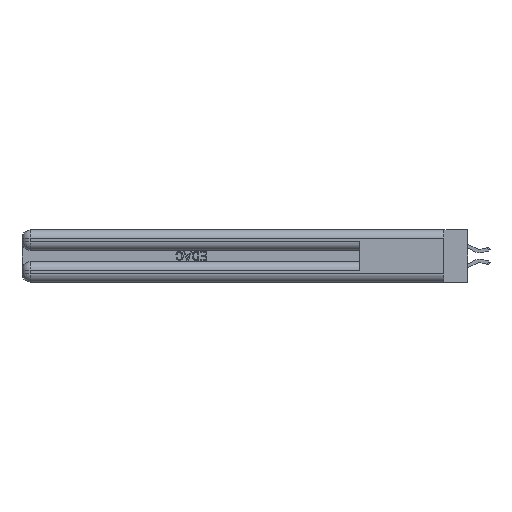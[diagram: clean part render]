
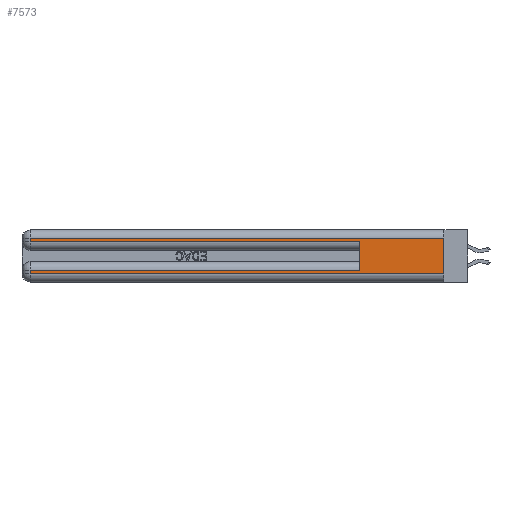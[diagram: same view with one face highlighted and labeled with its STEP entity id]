
A CAD part, left-side view. The second image highlights one B-rep face of the part: STEP entity #7573.
In plain terms, the highlighted planar face has unit normal (-1, 0, 0).
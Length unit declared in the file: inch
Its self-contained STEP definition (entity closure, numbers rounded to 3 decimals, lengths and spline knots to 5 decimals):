
#94 = ORIENTED_EDGE ( 'NONE', *, *, #21787, .T. ) ;
#700 = LINE ( 'NONE', #4594, #24358 ) ;
#827 = VECTOR ( 'NONE', #29109, 39.37008 ) ;
#887 = LINE ( 'NONE', #9848, #32662 ) ;
#1129 = DIRECTION ( 'NONE',  ( 0., 0., -1. ) ) ;
#2692 = VECTOR ( 'NONE', #24863, 39.37008 ) ;
#2916 = CARTESIAN_POINT ( 'NONE',  ( 0., 2.94, 0.06 ) ) ;
#3973 = ORIENTED_EDGE ( 'NONE', *, *, #18738, .T. ) ;
#4173 = ORIENTED_EDGE ( 'NONE', *, *, #19369, .F. ) ;
#4196 = EDGE_CURVE ( 'NONE', #21924, #30802, #9040, .T. ) ;
#4594 = CARTESIAN_POINT ( 'NONE',  ( 0., 2.94, 0.37 ) ) ;
#5489 = FACE_OUTER_BOUND ( 'NONE', #25918, .T. ) ;
#5833 = DIRECTION ( 'NONE',  ( 0., 0., -1. ) ) ;
#6884 = DIRECTION ( 'NONE',  ( 0., -1., 0. ) ) ;
#7479 = ORIENTED_EDGE ( 'NONE', *, *, #28998, .T. ) ;
#7573 = ADVANCED_FACE ( 'NONE', ( #5489 ), #18137, .F. ) ;
#8878 = VERTEX_POINT ( 'NONE', #20300 ) ;
#9040 = LINE ( 'NONE', #38211, #827 ) ;
#9848 = CARTESIAN_POINT ( 'NONE',  ( 0., 0., 0.285 ) ) ;
#11022 = ORIENTED_EDGE ( 'NONE', *, *, #28021, .T. ) ;
#13394 = CARTESIAN_POINT ( 'NONE',  ( 0., 2.94, 0.37 ) ) ;
#13627 = ORIENTED_EDGE ( 'NONE', *, *, #23504, .F. ) ;
#14803 = CARTESIAN_POINT ( 'NONE',  ( 0., 0.6, 0.085 ) ) ;
#15945 = EDGE_CURVE ( 'NONE', #8878, #22578, #887, .T. ) ;
#16010 = CARTESIAN_POINT ( 'NONE',  ( 0., 0., 0.085 ) ) ;
#17410 = CARTESIAN_POINT ( 'NONE',  ( 0., 2.94, 0.085 ) ) ;
#17546 = CARTESIAN_POINT ( 'NONE',  ( 0., 0., 0.06 ) ) ;
#17907 = VERTEX_POINT ( 'NONE', #14803 ) ;
#18137 = PLANE ( 'NONE',  #28725 ) ;
#18500 = DIRECTION ( 'NONE',  ( 0., 0., -1. ) ) ;
#18738 = EDGE_CURVE ( 'NONE', #35639, #34680, #20044, .T. ) ;
#19369 = EDGE_CURVE ( 'NONE', #21924, #34680, #22405, .T. ) ;
#19957 = DIRECTION ( 'NONE',  ( 0., 0., -1. ) ) ;
#20044 = LINE ( 'NONE', #33948, #2692 ) ;
#20300 = CARTESIAN_POINT ( 'NONE',  ( 0., 2.94, 0.285 ) ) ;
#21072 = CARTESIAN_POINT ( 'NONE',  ( 0., 2.94, 0.31 ) ) ;
#21211 = CARTESIAN_POINT ( 'NONE',  ( 0., 0., 0.37 ) ) ;
#21424 = DIRECTION ( 'NONE',  ( 0., 0., 1. ) ) ;
#21787 = EDGE_CURVE ( 'NONE', #17907, #24558, #34652, .T. ) ;
#21924 = VERTEX_POINT ( 'NONE', #32220 ) ;
#22405 = LINE ( 'NONE', #24544, #37739 ) ;
#22578 = VERTEX_POINT ( 'NONE', #22970 ) ;
#22970 = CARTESIAN_POINT ( 'NONE',  ( 0., 0.6, 0.285 ) ) ;
#23504 = EDGE_CURVE ( 'NONE', #17907, #22578, #26452, .T. ) ;
#24301 = DIRECTION ( 'NONE',  ( 1., 0., 0. ) ) ;
#24358 = VECTOR ( 'NONE', #19957, 39.37008 ) ;
#24544 = CARTESIAN_POINT ( 'NONE',  ( 0., 0., 0.37 ) ) ;
#24558 = VERTEX_POINT ( 'NONE', #17410 ) ;
#24863 = DIRECTION ( 'NONE',  ( 0., -1., 0. ) ) ;
#25918 = EDGE_LOOP ( 'NONE', ( #4173, #33603, #7479, #29957, #13627, #94, #11022, #3973 ) ) ;
#26452 = LINE ( 'NONE', #27469, #33655 ) ;
#26523 = VECTOR ( 'NONE', #37462, 39.37008 ) ;
#27469 = CARTESIAN_POINT ( 'NONE',  ( 0., 0.6, 0.145 ) ) ;
#28021 = EDGE_CURVE ( 'NONE', #24558, #35639, #700, .T. ) ;
#28725 = AXIS2_PLACEMENT_3D ( 'NONE', #21211, #24301, #5833 ) ;
#28998 = EDGE_CURVE ( 'NONE', #30802, #8878, #38194, .T. ) ;
#29109 = DIRECTION ( 'NONE',  ( 0., 1., 0. ) ) ;
#29957 = ORIENTED_EDGE ( 'NONE', *, *, #15945, .T. ) ;
#30802 = VERTEX_POINT ( 'NONE', #21072 ) ;
#32220 = CARTESIAN_POINT ( 'NONE',  ( 0., 0., 0.31 ) ) ;
#32662 = VECTOR ( 'NONE', #6884, 39.37008 ) ;
#33603 = ORIENTED_EDGE ( 'NONE', *, *, #4196, .T. ) ;
#33655 = VECTOR ( 'NONE', #21424, 39.37008 ) ;
#33948 = CARTESIAN_POINT ( 'NONE',  ( 0., 0., 0.06 ) ) ;
#34652 = LINE ( 'NONE', #16010, #26523 ) ;
#34680 = VERTEX_POINT ( 'NONE', #17546 ) ;
#35639 = VERTEX_POINT ( 'NONE', #2916 ) ;
#37236 = VECTOR ( 'NONE', #1129, 39.37008 ) ;
#37462 = DIRECTION ( 'NONE',  ( 0., 1., 0. ) ) ;
#37739 = VECTOR ( 'NONE', #18500, 39.37008 ) ;
#38194 = LINE ( 'NONE', #13394, #37236 ) ;
#38211 = CARTESIAN_POINT ( 'NONE',  ( 0., 0., 0.31 ) ) ;
